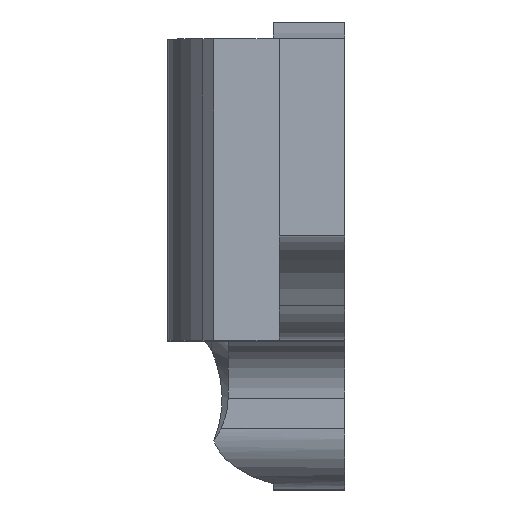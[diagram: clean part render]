
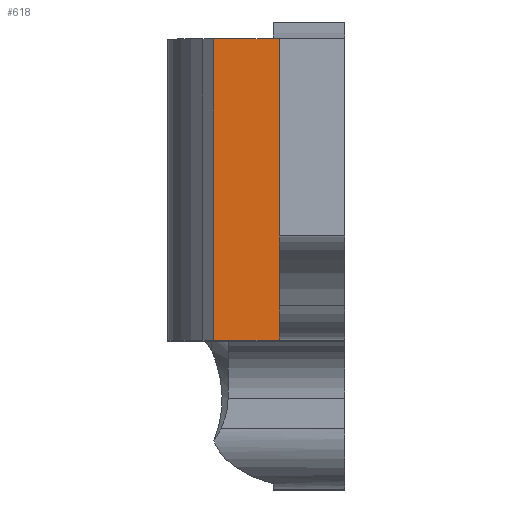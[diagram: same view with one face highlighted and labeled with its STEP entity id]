
A CAD part, top view. The second image highlights one B-rep face of the part: STEP entity #618.
In plain terms, the highlighted planar face has unit normal (0, 0, 1).
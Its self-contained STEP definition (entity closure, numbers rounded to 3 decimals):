
#39 = CARTESIAN_POINT ( 'NONE',  ( -18.407, -2.905, 114.976 ) ) ;
#63 = CARTESIAN_POINT ( 'NONE',  ( -15.17, -2.905, 114.976 ) ) ;
#80 = AXIS2_PLACEMENT_3D ( 'NONE', #538, #215, #542 ) ;
#215 = DIRECTION ( 'NONE',  ( 0., 0., 1. ) ) ;
#230 = EDGE_CURVE ( 'NONE', #1138, #1163, #1171, .T. ) ;
#231 = DIRECTION ( 'NONE',  ( 0., 1., 0. ) ) ;
#241 = FACE_OUTER_BOUND ( 'NONE', #1084, .T. ) ;
#366 = CARTESIAN_POINT ( 'NONE',  ( -18.407, -8.425, 114.976 ) ) ;
#386 = ORIENTED_EDGE ( 'NONE', *, *, #413, .F. ) ;
#389 = CARTESIAN_POINT ( 'NONE',  ( -20.69, -8.425, 114.976 ) ) ;
#398 = CARTESIAN_POINT ( 'NONE',  ( -37.28, -23.305, 114.976 ) ) ;
#413 = EDGE_CURVE ( 'NONE', #1163, #1286, #857, .T. ) ;
#450 = DIRECTION ( 'NONE',  ( 0., -1., 0. ) ) ;
#538 = CARTESIAN_POINT ( 'NONE',  ( -20.69, -2.905, 114.976 ) ) ;
#542 = DIRECTION ( 'NONE',  ( 0., -1., 0. ) ) ;
#550 = CARTESIAN_POINT ( 'NONE',  ( -18.407, -23.305, 114.976 ) ) ;
#573 = DIRECTION ( 'NONE',  ( 1., 0., 0. ) ) ;
#576 = DIRECTION ( 'NONE',  ( 1., 0., 0. ) ) ;
#580 = ORIENTED_EDGE ( 'NONE', *, *, #1275, .T. ) ;
#618 = ADVANCED_FACE ( 'NONE', ( #241 ), #1155, .T. ) ;
#723 = VERTEX_POINT ( 'NONE', #1302 ) ;
#857 = LINE ( 'NONE', #389, #1089 ) ;
#865 = VECTOR ( 'NONE', #231, 1000. ) ;
#887 = VECTOR ( 'NONE', #576, 1000. ) ;
#908 = CARTESIAN_POINT ( 'NONE',  ( -15.17, -8.425, 114.976 ) ) ;
#981 = LINE ( 'NONE', #63, #1132 ) ;
#1084 = EDGE_LOOP ( 'NONE', ( #1233, #580, #1258, #386 ) ) ;
#1089 = VECTOR ( 'NONE', #573, 1000. ) ;
#1128 = LINE ( 'NONE', #398, #887 ) ;
#1132 = VECTOR ( 'NONE', #450, 1000. ) ;
#1138 = VERTEX_POINT ( 'NONE', #550 ) ;
#1153 = EDGE_CURVE ( 'NONE', #1286, #723, #981, .T. ) ;
#1155 = PLANE ( 'NONE',  #80 ) ;
#1163 = VERTEX_POINT ( 'NONE', #366 ) ;
#1171 = LINE ( 'NONE', #39, #865 ) ;
#1233 = ORIENTED_EDGE ( 'NONE', *, *, #230, .F. ) ;
#1258 = ORIENTED_EDGE ( 'NONE', *, *, #1153, .F. ) ;
#1275 = EDGE_CURVE ( 'NONE', #1138, #723, #1128, .T. ) ;
#1286 = VERTEX_POINT ( 'NONE', #908 ) ;
#1302 = CARTESIAN_POINT ( 'NONE',  ( -15.17, -23.305, 114.976 ) ) ;
